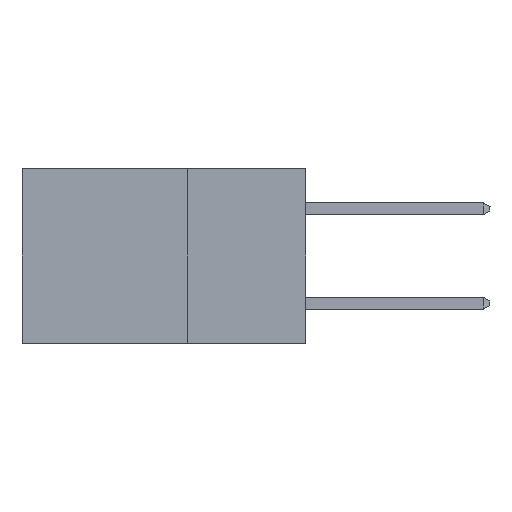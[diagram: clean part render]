
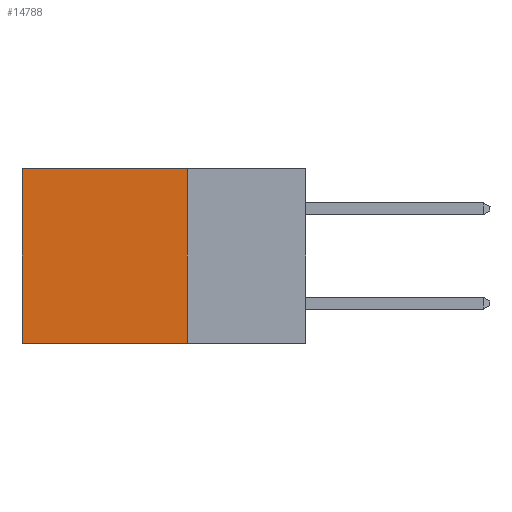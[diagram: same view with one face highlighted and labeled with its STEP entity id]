
A CAD part, left-side view. The second image highlights one B-rep face of the part: STEP entity #14788.
In plain terms, the highlighted planar face has unit normal (-1, 0, 0).
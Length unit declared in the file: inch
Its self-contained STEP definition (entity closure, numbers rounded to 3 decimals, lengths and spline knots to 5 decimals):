
#925 = CARTESIAN_POINT ( 'NONE',  ( 0.298, 0.25, 0. ) ) ;
#2047 = PLANE ( 'NONE',  #23291 ) ;
#2274 = CARTESIAN_POINT ( 'NONE',  ( 0.298, 0.25, 0. ) ) ;
#2406 = LINE ( 'NONE', #21976, #8367 ) ;
#3417 = VERTEX_POINT ( 'NONE', #7784 ) ;
#4806 = ORIENTED_EDGE ( 'NONE', *, *, #20264, .T. ) ;
#4854 = DIRECTION ( 'NONE',  ( 0., 0., -1. ) ) ;
#6123 = CARTESIAN_POINT ( 'NONE',  ( 0.298, 0.6, 0. ) ) ;
#6228 = ORIENTED_EDGE ( 'NONE', *, *, #22432, .F. ) ;
#7784 = CARTESIAN_POINT ( 'NONE',  ( 0.298, 0.6, -0.37 ) ) ;
#8367 = VECTOR ( 'NONE', #29581, 39.37008 ) ;
#8774 = VERTEX_POINT ( 'NONE', #6123 ) ;
#8997 = ORIENTED_EDGE ( 'NONE', *, *, #25725, .F. ) ;
#10916 = LINE ( 'NONE', #925, #24225 ) ;
#10987 = DIRECTION ( 'NONE',  ( 0., 0., -1. ) ) ;
#11266 = EDGE_CURVE ( 'NONE', #8774, #3417, #2406, .T. ) ;
#11659 = VERTEX_POINT ( 'NONE', #26352 ) ;
#12274 = CARTESIAN_POINT ( 'NONE',  ( 0.298, 0.25, -0.37 ) ) ;
#14788 = ADVANCED_FACE ( 'NONE', ( #28139 ), #2047, .F. ) ;
#17627 = ORIENTED_EDGE ( 'NONE', *, *, #11266, .T. ) ;
#18283 = VECTOR ( 'NONE', #27995, 39.37008 ) ;
#18614 = CARTESIAN_POINT ( 'NONE',  ( 0.298, 0.25, -0.37 ) ) ;
#19801 = LINE ( 'NONE', #18614, #25669 ) ;
#19907 = DIRECTION ( 'NONE',  ( 1., 0., 0. ) ) ;
#20264 = EDGE_CURVE ( 'NONE', #11659, #8774, #24901, .T. ) ;
#20422 = CARTESIAN_POINT ( 'NONE',  ( 0.298, 0.25, 0. ) ) ;
#21110 = DIRECTION ( 'NONE',  ( 0., 1., 0. ) ) ;
#21976 = CARTESIAN_POINT ( 'NONE',  ( 0.298, 0.6, 0. ) ) ;
#22432 = EDGE_CURVE ( 'NONE', #26078, #3417, #19801, .T. ) ;
#23291 = AXIS2_PLACEMENT_3D ( 'NONE', #2274, #19907, #4854 ) ;
#24225 = VECTOR ( 'NONE', #10987, 39.37008 ) ;
#24901 = LINE ( 'NONE', #20422, #18283 ) ;
#25669 = VECTOR ( 'NONE', #21110, 39.37008 ) ;
#25725 = EDGE_CURVE ( 'NONE', #11659, #26078, #10916, .T. ) ;
#26078 = VERTEX_POINT ( 'NONE', #12274 ) ;
#26352 = CARTESIAN_POINT ( 'NONE',  ( 0.298, 0.25, 0. ) ) ;
#27282 = EDGE_LOOP ( 'NONE', ( #17627, #6228, #8997, #4806 ) ) ;
#27995 = DIRECTION ( 'NONE',  ( 0., 1., 0. ) ) ;
#28139 = FACE_OUTER_BOUND ( 'NONE', #27282, .T. ) ;
#29581 = DIRECTION ( 'NONE',  ( 0., 0., -1. ) ) ;
